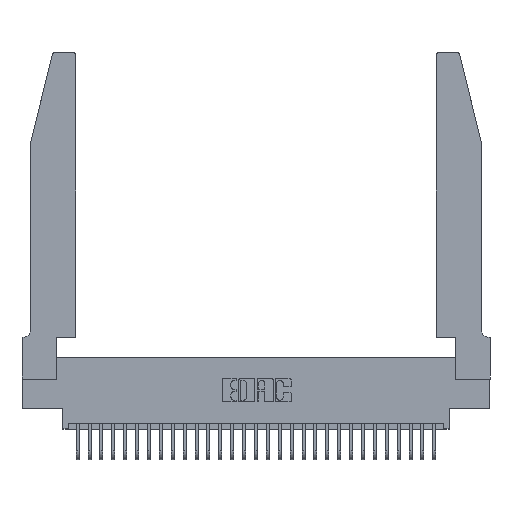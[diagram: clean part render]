
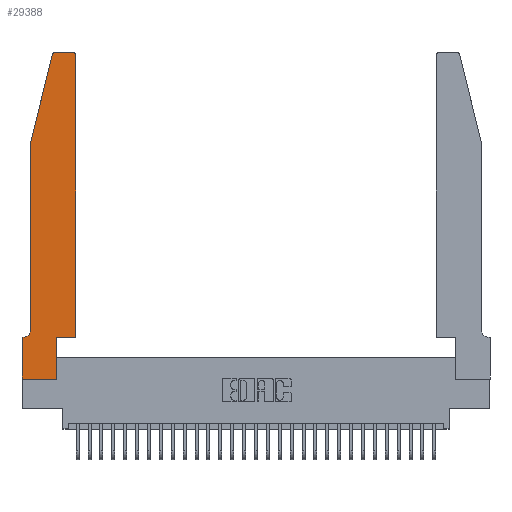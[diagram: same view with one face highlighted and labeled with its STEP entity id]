
A CAD part, top view. The second image highlights one B-rep face of the part: STEP entity #29388.
In plain terms, the highlighted planar face has unit normal (0, 0, 1).
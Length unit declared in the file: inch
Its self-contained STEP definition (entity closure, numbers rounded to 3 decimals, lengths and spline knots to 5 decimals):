
#389 = DIRECTION ( 'NONE',  ( -1., 0., 0. ) ) ;
#454 = VECTOR ( 'NONE', #389, 39.37008 ) ;
#460 = CARTESIAN_POINT ( 'NONE',  ( 0., 0., 0.37 ) ) ;
#729 = DIRECTION ( 'NONE',  ( 0., 1., 0. ) ) ;
#872 = CARTESIAN_POINT ( 'NONE',  ( 0.25487, 2.72718, 0.37 ) ) ;
#951 = VERTEX_POINT ( 'NONE', #460 ) ;
#1171 = ORIENTED_EDGE ( 'NONE', *, *, #1711, .T. ) ;
#1370 = DIRECTION ( 'NONE',  ( 1., 0., 0. ) ) ;
#1711 = EDGE_CURVE ( 'NONE', #20986, #24703, #21595, .T. ) ;
#1809 = CARTESIAN_POINT ( 'NONE',  ( 0., 0.35, 0.37 ) ) ;
#1841 = CARTESIAN_POINT ( 'NONE',  ( 0.4505, 0.35, 0.37 ) ) ;
#1892 = ORIENTED_EDGE ( 'NONE', *, *, #22291, .T. ) ;
#2251 = ORIENTED_EDGE ( 'NONE', *, *, #10113, .T. ) ;
#2628 = EDGE_CURVE ( 'NONE', #24836, #12504, #3848, .T. ) ;
#2679 = AXIS2_PLACEMENT_3D ( 'NONE', #6133, #22211, #8494 ) ;
#2856 = CIRCLE ( 'NONE', #3659, 0.03 ) ;
#3157 = VECTOR ( 'NONE', #729, 39.37008 ) ;
#3645 = EDGE_CURVE ( 'NONE', #29172, #8269, #24991, .T. ) ;
#3659 = AXIS2_PLACEMENT_3D ( 'NONE', #28894, #15427, #1370 ) ;
#3806 = AXIS2_PLACEMENT_3D ( 'NONE', #20138, #6280, #22348 ) ;
#3820 = CARTESIAN_POINT ( 'NONE',  ( 0.2605, 2.75, 0.37 ) ) ;
#3848 = LINE ( 'NONE', #22982, #21540 ) ;
#4319 = DIRECTION ( 'NONE',  ( 1., 0., 0. ) ) ;
#4378 = EDGE_CURVE ( 'NONE', #21360, #24836, #21559, .T. ) ;
#4411 = VECTOR ( 'NONE', #17153, 39.37008 ) ;
#5057 = CARTESIAN_POINT ( 'NONE',  ( 0., 0.35, 0.37 ) ) ;
#5428 = CARTESIAN_POINT ( 'NONE',  ( 0.4505, 0.35, 0.37 ) ) ;
#5998 = EDGE_CURVE ( 'NONE', #18468, #27609, #16834, .T. ) ;
#6133 = CARTESIAN_POINT ( 'NONE',  ( 0.0055, 0.42, 0.37 ) ) ;
#6280 = DIRECTION ( 'NONE',  ( 0., 0., 1. ) ) ;
#6329 = EDGE_LOOP ( 'NONE', ( #10629, #8826, #7711, #18990, #17262, #21723, #20717, #1892, #19341, #2251, #1171, #23168 ) ) ;
#6873 = DIRECTION ( 'NONE',  ( -0.239, -0.971, 0. ) ) ;
#7403 = DIRECTION ( 'NONE',  ( 0., 0., 1. ) ) ;
#7711 = ORIENTED_EDGE ( 'NONE', *, *, #4378, .T. ) ;
#8269 = VERTEX_POINT ( 'NONE', #1809 ) ;
#8494 = DIRECTION ( 'NONE',  ( -1., 0., 0. ) ) ;
#8826 = ORIENTED_EDGE ( 'NONE', *, *, #28492, .T. ) ;
#8902 = CARTESIAN_POINT ( 'NONE',  ( 0.2865, 0.35, 0.37 ) ) ;
#8963 = VERTEX_POINT ( 'NONE', #11280 ) ;
#9255 = EDGE_CURVE ( 'NONE', #8963, #14069, #28279, .T. ) ;
#10044 = VECTOR ( 'NONE', #22990, 39.37008 ) ;
#10090 = VECTOR ( 'NONE', #6873, 39.37008 ) ;
#10113 = EDGE_CURVE ( 'NONE', #27609, #20986, #16292, .T. ) ;
#10184 = CARTESIAN_POINT ( 'NONE',  ( 0.2865, 0.35, 0.37 ) ) ;
#10629 = ORIENTED_EDGE ( 'NONE', *, *, #9255, .T. ) ;
#10785 = CIRCLE ( 'NONE', #2679, 0.07 ) ;
#11103 = DIRECTION ( 'NONE',  ( 0., -1., 0. ) ) ;
#11280 = CARTESIAN_POINT ( 'NONE',  ( 0.4205, 2.75, 0.37 ) ) ;
#12078 = CARTESIAN_POINT ( 'NONE',  ( 0.0755, 0.35, 0.37 ) ) ;
#12442 = CARTESIAN_POINT ( 'NONE',  ( 0.4505, 2.72, 0.37 ) ) ;
#12504 = VERTEX_POINT ( 'NONE', #14649 ) ;
#12755 = EDGE_CURVE ( 'NONE', #12504, #29172, #10785, .T. ) ;
#14069 = VERTEX_POINT ( 'NONE', #24402 ) ;
#14649 = CARTESIAN_POINT ( 'NONE',  ( 0.0755, 0.42, 0.37 ) ) ;
#15427 = DIRECTION ( 'NONE',  ( 0., 0., 1. ) ) ;
#15967 = CARTESIAN_POINT ( 'NONE',  ( 0.0055, 0.35, 0.37 ) ) ;
#16292 = LINE ( 'NONE', #29713, #10044 ) ;
#16834 = LINE ( 'NONE', #10184, #4411 ) ;
#17153 = DIRECTION ( 'NONE',  ( 0., 1., 0. ) ) ;
#17262 = ORIENTED_EDGE ( 'NONE', *, *, #12755, .T. ) ;
#17346 = VECTOR ( 'NONE', #11103, 39.37008 ) ;
#18268 = EDGE_CURVE ( 'NONE', #8269, #951, #29277, .T. ) ;
#18273 = CARTESIAN_POINT ( 'NONE',  ( 0., 0., 0.37 ) ) ;
#18468 = VERTEX_POINT ( 'NONE', #26009 ) ;
#18489 = CARTESIAN_POINT ( 'NONE',  ( 0.0755, 2., 0.37 ) ) ;
#18989 = PLANE ( 'NONE',  #19631 ) ;
#18990 = ORIENTED_EDGE ( 'NONE', *, *, #2628, .T. ) ;
#19341 = ORIENTED_EDGE ( 'NONE', *, *, #5998, .T. ) ;
#19631 = AXIS2_PLACEMENT_3D ( 'NONE', #5057, #7403, #23441 ) ;
#19843 = CARTESIAN_POINT ( 'NONE',  ( 0.0755, 2., 0.37 ) ) ;
#20138 = CARTESIAN_POINT ( 'NONE',  ( 0.4205, 2.72, 0.37 ) ) ;
#20578 = FACE_OUTER_BOUND ( 'NONE', #6329, .T. ) ;
#20717 = ORIENTED_EDGE ( 'NONE', *, *, #18268, .T. ) ;
#20986 = VERTEX_POINT ( 'NONE', #1841 ) ;
#21295 = VECTOR ( 'NONE', #4319, 39.37008 ) ;
#21360 = VERTEX_POINT ( 'NONE', #872 ) ;
#21540 = VECTOR ( 'NONE', #23072, 39.37008 ) ;
#21559 = LINE ( 'NONE', #18489, #10090 ) ;
#21595 = LINE ( 'NONE', #5428, #3157 ) ;
#21723 = ORIENTED_EDGE ( 'NONE', *, *, #3645, .T. ) ;
#21987 = LINE ( 'NONE', #18273, #21295 ) ;
#22211 = DIRECTION ( 'NONE',  ( 0., 0., -1. ) ) ;
#22262 = VECTOR ( 'NONE', #26838, 39.37008 ) ;
#22291 = EDGE_CURVE ( 'NONE', #951, #18468, #21987, .T. ) ;
#22348 = DIRECTION ( 'NONE',  ( 1., 0., 0. ) ) ;
#22459 = CARTESIAN_POINT ( 'NONE',  ( 0., 0., 0.37 ) ) ;
#22536 = CIRCLE ( 'NONE', #3806, 0.03 ) ;
#22982 = CARTESIAN_POINT ( 'NONE',  ( 0.0755, 2., 0.37 ) ) ;
#22990 = DIRECTION ( 'NONE',  ( 1., 0., 0. ) ) ;
#23072 = DIRECTION ( 'NONE',  ( 0., -1., 0. ) ) ;
#23168 = ORIENTED_EDGE ( 'NONE', *, *, #24895, .T. ) ;
#23441 = DIRECTION ( 'NONE',  ( 1., 0., 0. ) ) ;
#24402 = CARTESIAN_POINT ( 'NONE',  ( 0.284, 2.75, 0.37 ) ) ;
#24703 = VERTEX_POINT ( 'NONE', #12442 ) ;
#24836 = VERTEX_POINT ( 'NONE', #19843 ) ;
#24895 = EDGE_CURVE ( 'NONE', #24703, #8963, #22536, .T. ) ;
#24991 = LINE ( 'NONE', #12078, #454 ) ;
#26009 = CARTESIAN_POINT ( 'NONE',  ( 0.2865, 0., 0.37 ) ) ;
#26838 = DIRECTION ( 'NONE',  ( -1., 0., 0. ) ) ;
#27609 = VERTEX_POINT ( 'NONE', #8902 ) ;
#28279 = LINE ( 'NONE', #3820, #22262 ) ;
#28492 = EDGE_CURVE ( 'NONE', #14069, #21360, #2856, .T. ) ;
#28894 = CARTESIAN_POINT ( 'NONE',  ( 0.284, 2.72, 0.37 ) ) ;
#29172 = VERTEX_POINT ( 'NONE', #15967 ) ;
#29277 = LINE ( 'NONE', #22459, #17346 ) ;
#29388 = ADVANCED_FACE ( 'NONE', ( #20578 ), #18989, .T. ) ;
#29713 = CARTESIAN_POINT ( 'NONE',  ( 0.4505, 0.35, 0.37 ) ) ;
